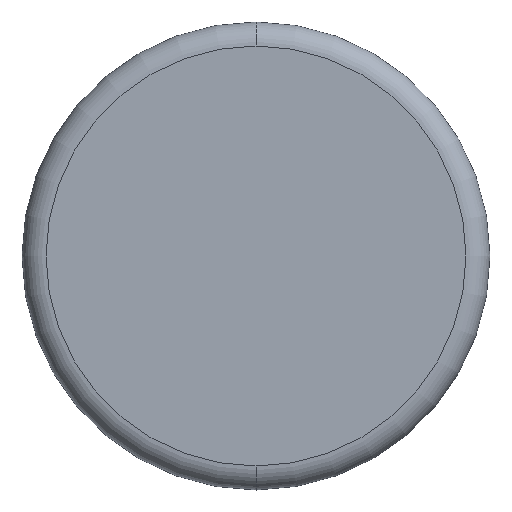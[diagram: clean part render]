
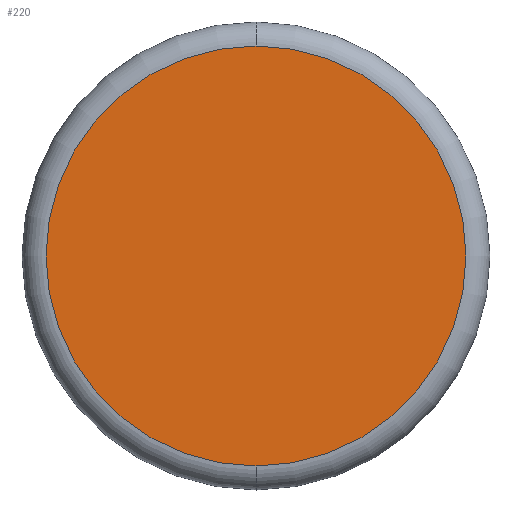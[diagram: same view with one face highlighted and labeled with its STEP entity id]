
A CAD part, front view. The second image highlights one B-rep face of the part: STEP entity #220.
In plain terms, the highlighted planar face has unit normal (0, -1, 0).
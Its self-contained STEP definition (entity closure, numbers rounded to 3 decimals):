
#25 = FACE_OUTER_BOUND ( 'NONE', #223, .T. ) ;
#39 = CIRCLE ( 'NONE', #273, 8.75 ) ;
#43 = CIRCLE ( 'NONE', #184, 8.75 ) ;
#87 = DIRECTION ( 'NONE',  ( 0., -1., 0. ) ) ;
#88 = DIRECTION ( 'NONE',  ( 0., 0., -1. ) ) ;
#102 = PLANE ( 'NONE',  #299 ) ;
#103 = DIRECTION ( 'NONE',  ( 0., -1., 0. ) ) ;
#105 = DIRECTION ( 'NONE',  ( 0., -1., 0. ) ) ;
#124 = CARTESIAN_POINT ( 'NONE',  ( 0., -2., 0. ) ) ;
#142 = EDGE_CURVE ( 'NONE', #265, #176, #43, .T. ) ;
#158 = CARTESIAN_POINT ( 'NONE',  ( 0., -2., 8.75 ) ) ;
#163 = ORIENTED_EDGE ( 'NONE', *, *, #172, .T. ) ;
#168 = ORIENTED_EDGE ( 'NONE', *, *, #142, .T. ) ;
#172 = EDGE_CURVE ( 'NONE', #176, #265, #39, .T. ) ;
#176 = VERTEX_POINT ( 'NONE', #301 ) ;
#184 = AXIS2_PLACEMENT_3D ( 'NONE', #279, #87, #248 ) ;
#220 = ADVANCED_FACE ( 'NONE', ( #25 ), #102, .T. ) ;
#223 = EDGE_LOOP ( 'NONE', ( #163, #168 ) ) ;
#248 = DIRECTION ( 'NONE',  ( 0., 0., -1. ) ) ;
#265 = VERTEX_POINT ( 'NONE', #158 ) ;
#273 = AXIS2_PLACEMENT_3D ( 'NONE', #298, #105, #278 ) ;
#278 = DIRECTION ( 'NONE',  ( 0., 0., -1. ) ) ;
#279 = CARTESIAN_POINT ( 'NONE',  ( 0., -2., 0. ) ) ;
#298 = CARTESIAN_POINT ( 'NONE',  ( 0., -2., 0. ) ) ;
#299 = AXIS2_PLACEMENT_3D ( 'NONE', #124, #103, #88 ) ;
#301 = CARTESIAN_POINT ( 'NONE',  ( 0., -2., -8.75 ) ) ;
